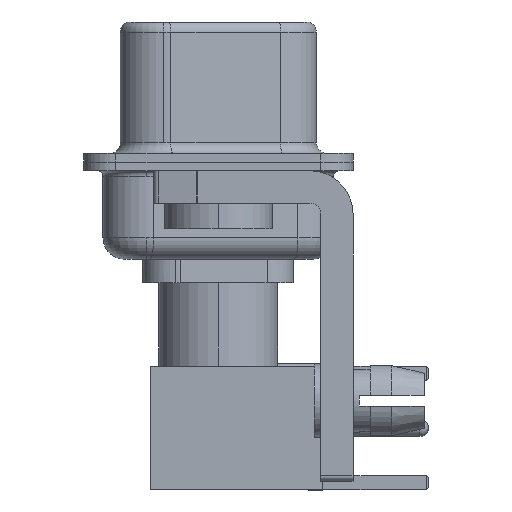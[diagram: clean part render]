
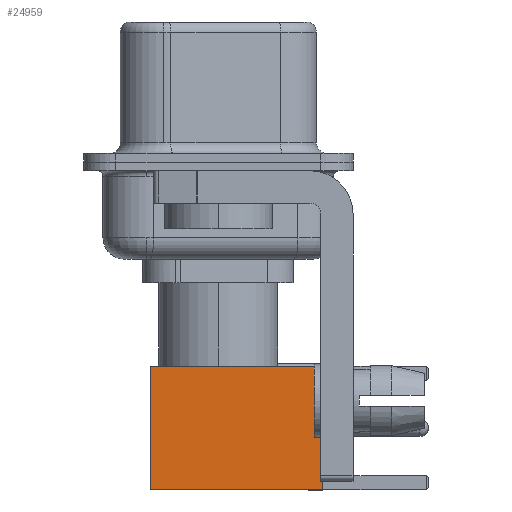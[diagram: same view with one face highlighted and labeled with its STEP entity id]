
A CAD part, left-side view. The second image highlights one B-rep face of the part: STEP entity #24959.
In plain terms, the highlighted face is planar.
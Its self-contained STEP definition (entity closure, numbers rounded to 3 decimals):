
#1097 = ORIENTED_EDGE ( 'NONE', *, *, #15837, .F. ) ;
#2120 = CARTESIAN_POINT ( 'NONE',  ( -2.875, 2.875, 0. ) ) ;
#2933 = ORIENTED_EDGE ( 'NONE', *, *, #6826, .T. ) ;
#3082 = CARTESIAN_POINT ( 'NONE',  ( -2.875, 2.875, 8. ) ) ;
#3902 = CARTESIAN_POINT ( 'NONE',  ( -2.875, 2.875, 0. ) ) ;
#4118 = ORIENTED_EDGE ( 'NONE', *, *, #8848, .F. ) ;
#4720 = VECTOR ( 'NONE', #24481, 1000. ) ;
#5691 = PLANE ( 'NONE',  #13895 ) ;
#6227 = VERTEX_POINT ( 'NONE', #8782 ) ;
#6369 = DIRECTION ( 'NONE',  ( 0., 0., -1. ) ) ;
#6826 = EDGE_CURVE ( 'NONE', #6227, #19713, #9866, .T. ) ;
#7263 = CARTESIAN_POINT ( 'NONE',  ( 2.875, 2.875, 0. ) ) ;
#7388 = FACE_OUTER_BOUND ( 'NONE', #27784, .T. ) ;
#8782 = CARTESIAN_POINT ( 'NONE',  ( 2.875, 2.875, 8. ) ) ;
#8848 = EDGE_CURVE ( 'NONE', #6227, #26166, #27654, .T. ) ;
#9633 = CARTESIAN_POINT ( 'NONE',  ( 2.875, 2.875, 0. ) ) ;
#9866 = LINE ( 'NONE', #20548, #4720 ) ;
#11509 = ORIENTED_EDGE ( 'NONE', *, *, #24455, .T. ) ;
#11821 = DIRECTION ( 'NONE',  ( -1., 0., 0. ) ) ;
#12384 = CARTESIAN_POINT ( 'NONE',  ( 0., 2.875, 8. ) ) ;
#13658 = LINE ( 'NONE', #20376, #21932 ) ;
#13895 = AXIS2_PLACEMENT_3D ( 'NONE', #9633, #24522, #16239 ) ;
#15837 = EDGE_CURVE ( 'NONE', #26166, #17040, #17323, .T. ) ;
#16239 = DIRECTION ( 'NONE',  ( 0., 0., 1. ) ) ;
#17040 = VERTEX_POINT ( 'NONE', #3902 ) ;
#17323 = LINE ( 'NONE', #2120, #21713 ) ;
#19713 = VERTEX_POINT ( 'NONE', #7263 ) ;
#20376 = CARTESIAN_POINT ( 'NONE',  ( 0., 2.875, 0. ) ) ;
#20548 = CARTESIAN_POINT ( 'NONE',  ( 2.875, 2.875, 0. ) ) ;
#20663 = VECTOR ( 'NONE', #20937, 1000. ) ;
#20937 = DIRECTION ( 'NONE',  ( -1., 0., 0. ) ) ;
#21713 = VECTOR ( 'NONE', #6369, 1000. ) ;
#21932 = VECTOR ( 'NONE', #11821, 1000. ) ;
#24455 = EDGE_CURVE ( 'NONE', #19713, #17040, #13658, .T. ) ;
#24481 = DIRECTION ( 'NONE',  ( 0., 0., -1. ) ) ;
#24522 = DIRECTION ( 'NONE',  ( 0., 1., 0. ) ) ;
#24959 = ADVANCED_FACE ( 'NONE', ( #7388 ), #5691, .T. ) ;
#26166 = VERTEX_POINT ( 'NONE', #3082 ) ;
#27654 = LINE ( 'NONE', #12384, #20663 ) ;
#27784 = EDGE_LOOP ( 'NONE', ( #2933, #11509, #1097, #4118 ) ) ;
